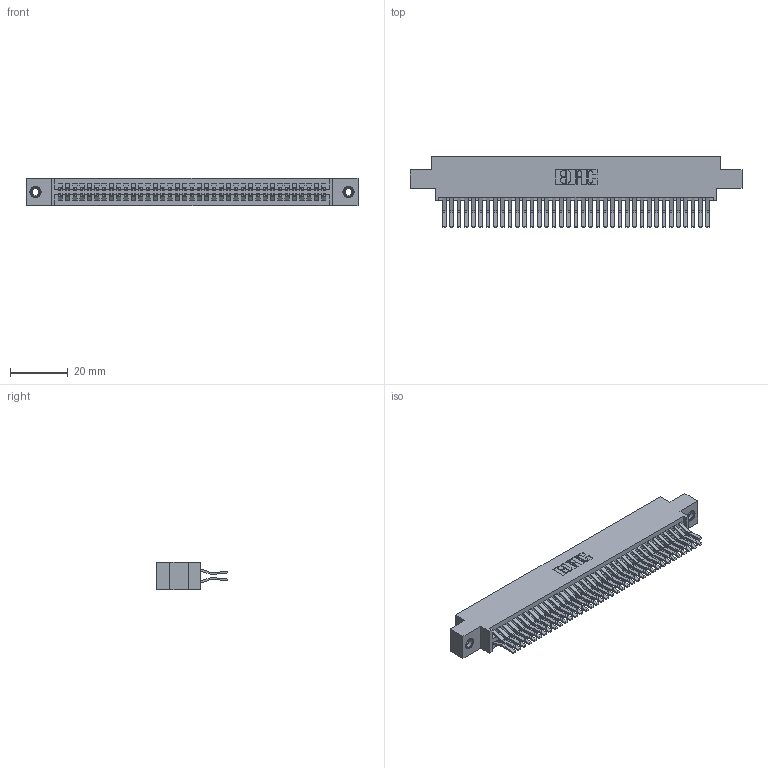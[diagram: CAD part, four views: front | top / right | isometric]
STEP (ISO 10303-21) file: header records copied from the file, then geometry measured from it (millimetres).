
FILE_DESCRIPTION (( 'STEP AP203' ), '1' );
FILE_NAME ('395-074-560-808.STEP', '2019-10-24T15:42:22', ( '' ), ( '' ), 'SwSTEP 2.0', 'SolidWorks 2016', '' );
FILE_SCHEMA (( 'CONFIG_CONTROL_DESIGN' ));
Length unit declared in the file: inch
Products named in the file (4): 345 Part_0.170 Offset - 0.156 Dia-TI; 345-292-001_560 Tail; 345-250-001_345-250-003-102; 395-074-560-808
Assembly tree (77 placements, depth 2):
  395-074-560-808
    345 Part_0.170 Offset - 0.156 Dia-TI
    345-292-001_560 Tail  x74
    345-250-001_345-250-003-102  x2
Bounding box: 115.19 x 24.45 x 9.4 mm (x, y, z)
Volume: 11508.3 mm3; surface area: 18318.7 mm2
Topology: 77 solids, 77 shells, 4038 faces, 11959 edges, 7866 vertices
Faces by surface type: plane 2558, cylinder 1464, cone 12, torus 4
Entity records: 31110 total; most frequent: CARTESIAN_POINT 5203, ORIENTED_EDGE 5130, DIRECTION 4623, EDGE_CURVE 2565, VECTOR 2261, LINE 2261, VERTEX_POINT 1704, AXIS2_PLACEMENT_3D 1181
